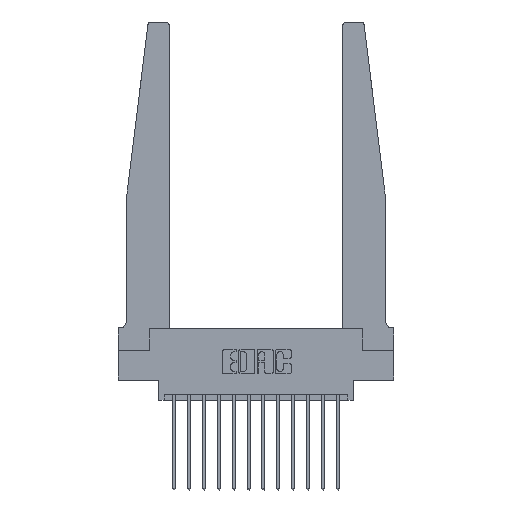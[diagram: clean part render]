
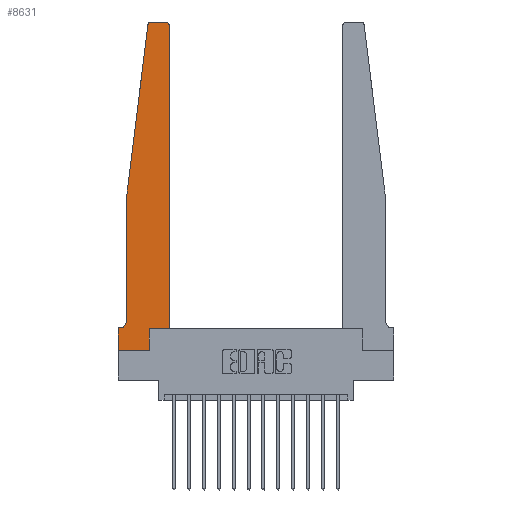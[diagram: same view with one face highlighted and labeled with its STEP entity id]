
A CAD part, top view. The second image highlights one B-rep face of the part: STEP entity #8631.
In plain terms, the highlighted planar face has unit normal (0, 0, 1).
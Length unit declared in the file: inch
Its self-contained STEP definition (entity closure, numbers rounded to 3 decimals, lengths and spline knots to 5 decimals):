
#64 = DIRECTION ( 'NONE',  ( 0., 0., -1. ) ) ;
#77 = VECTOR ( 'NONE', #5807, 39.37008 ) ;
#531 = DIRECTION ( 'NONE',  ( 1., 0., 0. ) ) ;
#793 = LINE ( 'NONE', #1997, #77 ) ;
#896 = CARTESIAN_POINT ( 'NONE',  ( 0.015, 0.1875, 0.37 ) ) ;
#1334 = AXIS2_PLACEMENT_3D ( 'NONE', #14644, #64, #4126 ) ;
#1340 = EDGE_CURVE ( 'NONE', #2046, #11710, #12387, .T. ) ;
#1650 = VECTOR ( 'NONE', #2341, 39.37008 ) ;
#1949 = VERTEX_POINT ( 'NONE', #13546 ) ;
#1997 = CARTESIAN_POINT ( 'NONE',  ( 0.425, 0.18, 0.37 ) ) ;
#2046 = VERTEX_POINT ( 'NONE', #9703 ) ;
#2096 = CARTESIAN_POINT ( 'NONE',  ( 0., 0.1875, 0.37 ) ) ;
#2244 = DIRECTION ( 'NONE',  ( 1., 0., 0. ) ) ;
#2250 = EDGE_LOOP ( 'NONE', ( #5314, #7312, #8218, #6228, #6504, #6488, #5084, #5925, #11367, #13427, #8633, #9212 ) ) ;
#2341 = DIRECTION ( 'NONE',  ( 0., -1., 0. ) ) ;
#2986 = VECTOR ( 'NONE', #15239, 39.37008 ) ;
#3124 = DIRECTION ( 'NONE',  ( 0., -1., 0. ) ) ;
#3274 = VECTOR ( 'NONE', #3124, 39.37008 ) ;
#3397 = CARTESIAN_POINT ( 'NONE',  ( 0.425, 2.72, 0.37 ) ) ;
#3587 = LINE ( 'NONE', #14163, #16858 ) ;
#3711 = DIRECTION ( 'NONE',  ( 1., 0., 0. ) ) ;
#4126 = DIRECTION ( 'NONE',  ( -1., 0., 0. ) ) ;
#4349 = CARTESIAN_POINT ( 'NONE',  ( 0., 0., 0.37 ) ) ;
#4381 = LINE ( 'NONE', #8740, #3274 ) ;
#4511 = CARTESIAN_POINT ( 'NONE',  ( 0.425, 0.18, 0.37 ) ) ;
#4559 = CARTESIAN_POINT ( 'NONE',  ( 0.395, 2.72, 0.37 ) ) ;
#4649 = AXIS2_PLACEMENT_3D ( 'NONE', #4559, #11249, #531 ) ;
#5084 = ORIENTED_EDGE ( 'NONE', *, *, #10417, .T. ) ;
#5314 = ORIENTED_EDGE ( 'NONE', *, *, #13287, .T. ) ;
#5343 = LINE ( 'NONE', #13958, #15229 ) ;
#5648 = EDGE_CURVE ( 'NONE', #10583, #12343, #793, .T. ) ;
#5746 = AXIS2_PLACEMENT_3D ( 'NONE', #2096, #6130, #3711 ) ;
#5807 = DIRECTION ( 'NONE',  ( 1., 0., 0. ) ) ;
#5847 = VERTEX_POINT ( 'NONE', #12872 ) ;
#5890 = EDGE_CURVE ( 'NONE', #9502, #5847, #14107, .T. ) ;
#5925 = ORIENTED_EDGE ( 'NONE', *, *, #12888, .T. ) ;
#5953 = CARTESIAN_POINT ( 'NONE',  ( 0.27653, 2.72, 0.37 ) ) ;
#5974 = DIRECTION ( 'NONE',  ( -1., 0., 0. ) ) ;
#6130 = DIRECTION ( 'NONE',  ( 0., 0., 1. ) ) ;
#6228 = ORIENTED_EDGE ( 'NONE', *, *, #6973, .T. ) ;
#6271 = CARTESIAN_POINT ( 'NONE',  ( 0.425, 0.18, 0.37 ) ) ;
#6488 = ORIENTED_EDGE ( 'NONE', *, *, #5890, .T. ) ;
#6504 = ORIENTED_EDGE ( 'NONE', *, *, #11397, .T. ) ;
#6787 = VERTEX_POINT ( 'NONE', #4349 ) ;
#6973 = EDGE_CURVE ( 'NONE', #12129, #9039, #11602, .T. ) ;
#7312 = ORIENTED_EDGE ( 'NONE', *, *, #1340, .T. ) ;
#7540 = CARTESIAN_POINT ( 'NONE',  ( 0.065, 0.1875, 0.37 ) ) ;
#7921 = VECTOR ( 'NONE', #12790, 39.37008 ) ;
#8218 = ORIENTED_EDGE ( 'NONE', *, *, #10393, .T. ) ;
#8631 = ADVANCED_FACE ( 'NONE', ( #9720 ), #11724, .T. ) ;
#8633 = ORIENTED_EDGE ( 'NONE', *, *, #10465, .T. ) ;
#8740 = CARTESIAN_POINT ( 'NONE',  ( 0., 0., 0.37 ) ) ;
#8773 = LINE ( 'NONE', #10061, #10766 ) ;
#9003 = CARTESIAN_POINT ( 'NONE',  ( 0.065, 1.25, 0.37 ) ) ;
#9039 = VERTEX_POINT ( 'NONE', #9330 ) ;
#9212 = ORIENTED_EDGE ( 'NONE', *, *, #13698, .T. ) ;
#9330 = CARTESIAN_POINT ( 'NONE',  ( 0.065, 0.2375, 0.37 ) ) ;
#9502 = VERTEX_POINT ( 'NONE', #896 ) ;
#9703 = CARTESIAN_POINT ( 'NONE',  ( 0.27653, 2.75, 0.37 ) ) ;
#9720 = FACE_OUTER_BOUND ( 'NONE', #2250, .T. ) ;
#10061 = CARTESIAN_POINT ( 'NONE',  ( 0.25, 2.75, 0.37 ) ) ;
#10393 = EDGE_CURVE ( 'NONE', #11710, #12129, #13668, .T. ) ;
#10417 = EDGE_CURVE ( 'NONE', #5847, #6787, #4381, .T. ) ;
#10465 = EDGE_CURVE ( 'NONE', #12343, #15428, #12489, .T. ) ;
#10583 = VERTEX_POINT ( 'NONE', #17087 ) ;
#10766 = VECTOR ( 'NONE', #5974, 39.37008 ) ;
#11249 = DIRECTION ( 'NONE',  ( 0., 0., 1. ) ) ;
#11367 = ORIENTED_EDGE ( 'NONE', *, *, #14037, .T. ) ;
#11397 = EDGE_CURVE ( 'NONE', #9039, #9502, #13299, .T. ) ;
#11427 = DIRECTION ( 'NONE',  ( 1., 0., 0. ) ) ;
#11602 = LINE ( 'NONE', #9003, #1650 ) ;
#11710 = VERTEX_POINT ( 'NONE', #15970 ) ;
#11724 = PLANE ( 'NONE',  #5746 ) ;
#11792 = CARTESIAN_POINT ( 'NONE',  ( 0.065, 1.25, 0.37 ) ) ;
#12129 = VERTEX_POINT ( 'NONE', #11792 ) ;
#12189 = VERTEX_POINT ( 'NONE', #16537 ) ;
#12343 = VERTEX_POINT ( 'NONE', #6271 ) ;
#12387 = CIRCLE ( 'NONE', #15737, 0.03 ) ;
#12489 = LINE ( 'NONE', #4511, #14089 ) ;
#12790 = DIRECTION ( 'NONE',  ( -1., 0., 0. ) ) ;
#12872 = CARTESIAN_POINT ( 'NONE',  ( 0., 0.1875, 0.37 ) ) ;
#12888 = EDGE_CURVE ( 'NONE', #6787, #1949, #3587, .T. ) ;
#12960 = CIRCLE ( 'NONE', #4649, 0.03 ) ;
#13287 = EDGE_CURVE ( 'NONE', #12189, #2046, #8773, .T. ) ;
#13299 = CIRCLE ( 'NONE', #1334, 0.05 ) ;
#13427 = ORIENTED_EDGE ( 'NONE', *, *, #5648, .T. ) ;
#13546 = CARTESIAN_POINT ( 'NONE',  ( 0.2605, 0., 0.37 ) ) ;
#13668 = LINE ( 'NONE', #15054, #2986 ) ;
#13698 = EDGE_CURVE ( 'NONE', #15428, #12189, #12960, .T. ) ;
#13958 = CARTESIAN_POINT ( 'NONE',  ( 0.2605, 0.18, 0.37 ) ) ;
#14037 = EDGE_CURVE ( 'NONE', #1949, #10583, #5343, .T. ) ;
#14089 = VECTOR ( 'NONE', #16667, 39.37008 ) ;
#14107 = LINE ( 'NONE', #7540, #7921 ) ;
#14163 = CARTESIAN_POINT ( 'NONE',  ( 0., 0., 0.37 ) ) ;
#14644 = CARTESIAN_POINT ( 'NONE',  ( 0.015, 0.2375, 0.37 ) ) ;
#15054 = CARTESIAN_POINT ( 'NONE',  ( 0.065, 1.25, 0.37 ) ) ;
#15229 = VECTOR ( 'NONE', #15936, 39.37008 ) ;
#15239 = DIRECTION ( 'NONE',  ( -0.122, -0.992, 0. ) ) ;
#15250 = DIRECTION ( 'NONE',  ( 0., 0., 1. ) ) ;
#15428 = VERTEX_POINT ( 'NONE', #3397 ) ;
#15737 = AXIS2_PLACEMENT_3D ( 'NONE', #5953, #15250, #11427 ) ;
#15936 = DIRECTION ( 'NONE',  ( 0., 1., 0. ) ) ;
#15970 = CARTESIAN_POINT ( 'NONE',  ( 0.24675, 2.72367, 0.37 ) ) ;
#16537 = CARTESIAN_POINT ( 'NONE',  ( 0.395, 2.75, 0.37 ) ) ;
#16667 = DIRECTION ( 'NONE',  ( 0., 1., 0. ) ) ;
#16858 = VECTOR ( 'NONE', #2244, 39.37008 ) ;
#17087 = CARTESIAN_POINT ( 'NONE',  ( 0.2605, 0.18, 0.37 ) ) ;
